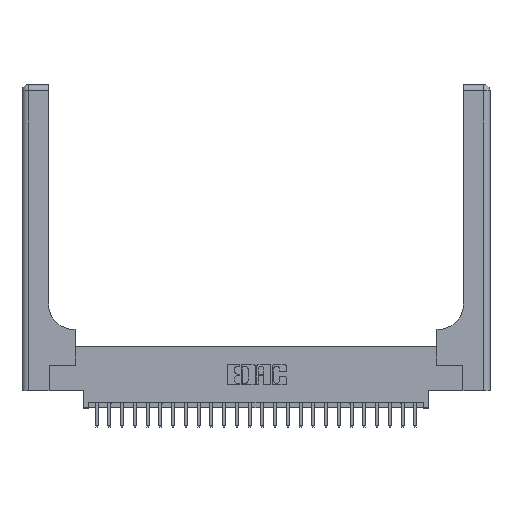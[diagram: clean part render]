
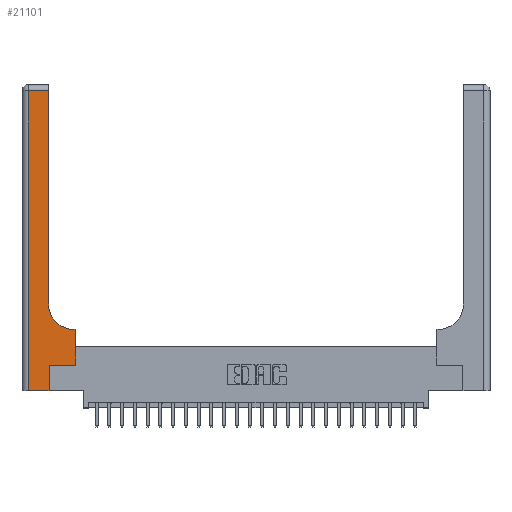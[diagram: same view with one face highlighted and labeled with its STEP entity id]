
A CAD part, top view. The second image highlights one B-rep face of the part: STEP entity #21101.
In plain terms, the highlighted planar face has unit normal (0, 0, 1).
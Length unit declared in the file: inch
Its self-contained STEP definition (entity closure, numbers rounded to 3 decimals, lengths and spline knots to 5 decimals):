
#30 = PLANE ( 'NONE',  #3421 ) ;
#892 = CARTESIAN_POINT ( 'NONE',  ( 0., 0., 0.37 ) ) ;
#1061 = CARTESIAN_POINT ( 'NONE',  ( 0., 2.94, 0.37 ) ) ;
#1716 = CARTESIAN_POINT ( 'NONE',  ( 0.51, 0.6, 0.37 ) ) ;
#2103 = CARTESIAN_POINT ( 'NONE',  ( 0.06, 2.94, 0.37 ) ) ;
#2520 = VERTEX_POINT ( 'NONE', #20498 ) ;
#2830 = EDGE_CURVE ( 'NONE', #19419, #19859, #14412, .T. ) ;
#3021 = DIRECTION ( 'NONE',  ( 0., 0., -1. ) ) ;
#3411 = ORIENTED_EDGE ( 'NONE', *, *, #19798, .T. ) ;
#3421 = AXIS2_PLACEMENT_3D ( 'NONE', #7827, #21094, #9739 ) ;
#3505 = LINE ( 'NONE', #1061, #13123 ) ;
#3511 = ORIENTED_EDGE ( 'NONE', *, *, #2830, .T. ) ;
#4010 = VECTOR ( 'NONE', #19303, 39.37008 ) ;
#4065 = ORIENTED_EDGE ( 'NONE', *, *, #16703, .T. ) ;
#4885 = EDGE_CURVE ( 'NONE', #2520, #19419, #22833, .T. ) ;
#5081 = EDGE_CURVE ( 'NONE', #17087, #8926, #3505, .T. ) ;
#5524 = DIRECTION ( 'NONE',  ( 0., 1., 0. ) ) ;
#6059 = LINE ( 'NONE', #9767, #16278 ) ;
#6309 = CARTESIAN_POINT ( 'NONE',  ( 0.265, 0.25, 0.37 ) ) ;
#7827 = CARTESIAN_POINT ( 'NONE',  ( 0., 3., 0.37 ) ) ;
#7917 = CARTESIAN_POINT ( 'NONE',  ( 0.06, 3., 0.37 ) ) ;
#8311 = CARTESIAN_POINT ( 'NONE',  ( 0.528, 0.25, 0.37 ) ) ;
#8565 = DIRECTION ( 'NONE',  ( 1., 0., 0. ) ) ;
#8926 = VERTEX_POINT ( 'NONE', #2103 ) ;
#8988 = CARTESIAN_POINT ( 'NONE',  ( 0.26, 2.94, 0.37 ) ) ;
#9113 = LINE ( 'NONE', #7917, #4010 ) ;
#9739 = DIRECTION ( 'NONE',  ( -1., 0., 0. ) ) ;
#9767 = CARTESIAN_POINT ( 'NONE',  ( 0.26, 0.6, 0.37 ) ) ;
#10570 = DIRECTION ( 'NONE',  ( 0., 1., 0. ) ) ;
#10649 = CARTESIAN_POINT ( 'NONE',  ( 0.528, 0.25, 0.37 ) ) ;
#10673 = ORIENTED_EDGE ( 'NONE', *, *, #4885, .T. ) ;
#11692 = DIRECTION ( 'NONE',  ( -1., 0., 0. ) ) ;
#12392 = VECTOR ( 'NONE', #5524, 39.37008 ) ;
#12663 = ORIENTED_EDGE ( 'NONE', *, *, #5081, .T. ) ;
#12738 = VECTOR ( 'NONE', #14778, 39.37008 ) ;
#12836 = CARTESIAN_POINT ( 'NONE',  ( 0.265, 0., 0.37 ) ) ;
#13088 = ORIENTED_EDGE ( 'NONE', *, *, #17031, .T. ) ;
#13123 = VECTOR ( 'NONE', #23804, 39.37008 ) ;
#13245 = CARTESIAN_POINT ( 'NONE',  ( 0.26, 3., 0.37 ) ) ;
#14054 = LINE ( 'NONE', #892, #20316 ) ;
#14248 = ORIENTED_EDGE ( 'NONE', *, *, #14885, .T. ) ;
#14412 = LINE ( 'NONE', #10649, #15607 ) ;
#14539 = CARTESIAN_POINT ( 'NONE',  ( 0.51, 0.85, 0.37 ) ) ;
#14760 = CARTESIAN_POINT ( 'NONE',  ( 0.26, 0.85, 0.37 ) ) ;
#14778 = DIRECTION ( 'NONE',  ( 0., 1., 0. ) ) ;
#14885 = EDGE_CURVE ( 'NONE', #18384, #2520, #18395, .T. ) ;
#15015 = EDGE_LOOP ( 'NONE', ( #3411, #12663, #17116, #18789, #14248, #10673, #3511, #4065, #13088 ) ) ;
#15567 = EDGE_CURVE ( 'NONE', #8926, #19743, #9113, .T. ) ;
#15607 = VECTOR ( 'NONE', #10570, 39.37008 ) ;
#15982 = VERTEX_POINT ( 'NONE', #1716 ) ;
#16278 = VECTOR ( 'NONE', #11692, 39.37008 ) ;
#16456 = DIRECTION ( 'NONE',  ( 1., 0., 0. ) ) ;
#16703 = EDGE_CURVE ( 'NONE', #19859, #15982, #6059, .T. ) ;
#17031 = EDGE_CURVE ( 'NONE', #15982, #17916, #24066, .T. ) ;
#17087 = VERTEX_POINT ( 'NONE', #8988 ) ;
#17116 = ORIENTED_EDGE ( 'NONE', *, *, #15567, .T. ) ;
#17468 = EDGE_CURVE ( 'NONE', #19743, #18384, #14054, .T. ) ;
#17762 = DIRECTION ( 'NONE',  ( 1., 0., 0. ) ) ;
#17916 = VERTEX_POINT ( 'NONE', #14760 ) ;
#18000 = FACE_OUTER_BOUND ( 'NONE', #15015, .T. ) ;
#18068 = LINE ( 'NONE', #13245, #12392 ) ;
#18384 = VERTEX_POINT ( 'NONE', #24168 ) ;
#18395 = LINE ( 'NONE', #12836, #12738 ) ;
#18588 = AXIS2_PLACEMENT_3D ( 'NONE', #14539, #3021, #16456 ) ;
#18789 = ORIENTED_EDGE ( 'NONE', *, *, #17468, .T. ) ;
#19037 = CARTESIAN_POINT ( 'NONE',  ( 0.528, 0.6, 0.37 ) ) ;
#19303 = DIRECTION ( 'NONE',  ( 0., -1., 0. ) ) ;
#19419 = VERTEX_POINT ( 'NONE', #8311 ) ;
#19743 = VERTEX_POINT ( 'NONE', #20671 ) ;
#19798 = EDGE_CURVE ( 'NONE', #17916, #17087, #18068, .T. ) ;
#19859 = VERTEX_POINT ( 'NONE', #19037 ) ;
#20316 = VECTOR ( 'NONE', #8565, 39.37008 ) ;
#20498 = CARTESIAN_POINT ( 'NONE',  ( 0.265, 0.25, 0.37 ) ) ;
#20671 = CARTESIAN_POINT ( 'NONE',  ( 0.06, 0., 0.37 ) ) ;
#21094 = DIRECTION ( 'NONE',  ( 0., 0., -1. ) ) ;
#21101 = ADVANCED_FACE ( 'NONE', ( #18000 ), #30, .F. ) ;
#22246 = VECTOR ( 'NONE', #17762, 39.37008 ) ;
#22833 = LINE ( 'NONE', #6309, #22246 ) ;
#23804 = DIRECTION ( 'NONE',  ( -1., 0., 0. ) ) ;
#24066 = CIRCLE ( 'NONE', #18588, 0.25 ) ;
#24168 = CARTESIAN_POINT ( 'NONE',  ( 0.265, 0., 0.37 ) ) ;
